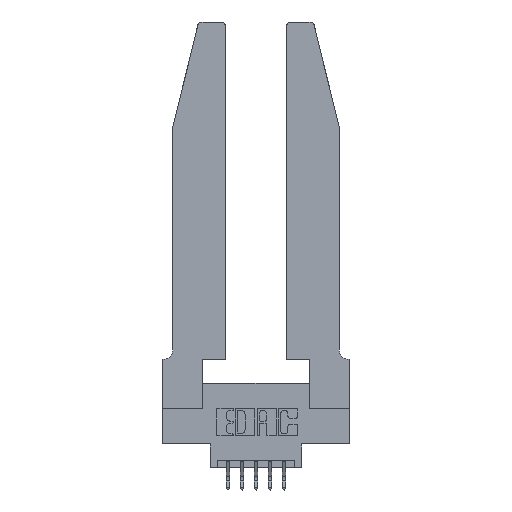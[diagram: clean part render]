
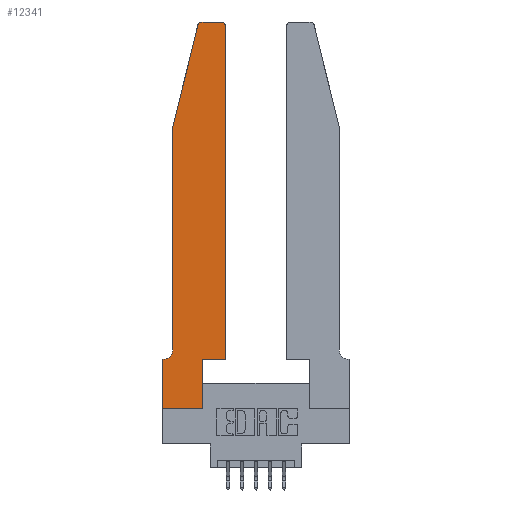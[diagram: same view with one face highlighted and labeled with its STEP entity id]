
A CAD part, top view. The second image highlights one B-rep face of the part: STEP entity #12341.
In plain terms, the highlighted planar face has unit normal (0, 0, 1).
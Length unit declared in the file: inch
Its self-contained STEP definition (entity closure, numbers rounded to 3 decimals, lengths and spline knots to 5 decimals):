
#237 = ORIENTED_EDGE ( 'NONE', *, *, #8766, .T. ) ;
#251 = ORIENTED_EDGE ( 'NONE', *, *, #8956, .T. ) ;
#315 = VERTEX_POINT ( 'NONE', #3736 ) ;
#317 = CARTESIAN_POINT ( 'NONE',  ( 0., 0.35, 0.37 ) ) ;
#403 = CARTESIAN_POINT ( 'NONE',  ( 0.0755, 0.35, 0.37 ) ) ;
#406 = DIRECTION ( 'NONE',  ( -1., 0., 0. ) ) ;
#435 = CARTESIAN_POINT ( 'NONE',  ( 0.4505, 2.72, 0.37 ) ) ;
#501 = CARTESIAN_POINT ( 'NONE',  ( 0., 0., 0.37 ) ) ;
#901 = ORIENTED_EDGE ( 'NONE', *, *, #8134, .T. ) ;
#904 = CARTESIAN_POINT ( 'NONE',  ( 0.0755, 2., 0.37 ) ) ;
#921 = LINE ( 'NONE', #1703, #2313 ) ;
#948 = AXIS2_PLACEMENT_3D ( 'NONE', #317, #1209, #2406 ) ;
#1146 = VERTEX_POINT ( 'NONE', #3767 ) ;
#1209 = DIRECTION ( 'NONE',  ( 0., 0., 1. ) ) ;
#1345 = EDGE_CURVE ( 'NONE', #9358, #4313, #7633, .T. ) ;
#1703 = CARTESIAN_POINT ( 'NONE',  ( 0.4505, 0.35, 0.37 ) ) ;
#1704 = DIRECTION ( 'NONE',  ( 1., 0., 0. ) ) ;
#1751 = DIRECTION ( 'NONE',  ( 0., 0., 1. ) ) ;
#1765 = CARTESIAN_POINT ( 'NONE',  ( 0., 0., 0.37 ) ) ;
#1826 = AXIS2_PLACEMENT_3D ( 'NONE', #13986, #12858, #11785 ) ;
#2122 = VERTEX_POINT ( 'NONE', #435 ) ;
#2232 = ORIENTED_EDGE ( 'NONE', *, *, #6194, .T. ) ;
#2313 = VECTOR ( 'NONE', #7273, 39.37008 ) ;
#2370 = CARTESIAN_POINT ( 'NONE',  ( 0.0755, 2., 0.37 ) ) ;
#2406 = DIRECTION ( 'NONE',  ( 1., 0., 0. ) ) ;
#2489 = CARTESIAN_POINT ( 'NONE',  ( 0.25487, 2.72718, 0.37 ) ) ;
#2533 = EDGE_CURVE ( 'NONE', #315, #7912, #9642, .T. ) ;
#2596 = DIRECTION ( 'NONE',  ( 0., 1., 0. ) ) ;
#2694 = CARTESIAN_POINT ( 'NONE',  ( 0.0055, 0.35, 0.37 ) ) ;
#2858 = DIRECTION ( 'NONE',  ( 0., 0., -1. ) ) ;
#2943 = CARTESIAN_POINT ( 'NONE',  ( 0.2865, 0., 0.37 ) ) ;
#3145 = CIRCLE ( 'NONE', #9103, 0.07 ) ;
#3296 = VECTOR ( 'NONE', #2596, 39.37008 ) ;
#3346 = ORIENTED_EDGE ( 'NONE', *, *, #8570, .T. ) ;
#3736 = CARTESIAN_POINT ( 'NONE',  ( 0.4205, 2.75, 0.37 ) ) ;
#3767 = CARTESIAN_POINT ( 'NONE',  ( 0.4505, 0.35, 0.37 ) ) ;
#3906 = VECTOR ( 'NONE', #5888, 39.37008 ) ;
#4260 = ORIENTED_EDGE ( 'NONE', *, *, #12443, .T. ) ;
#4313 = VERTEX_POINT ( 'NONE', #904 ) ;
#4517 = ORIENTED_EDGE ( 'NONE', *, *, #1345, .T. ) ;
#4708 = CARTESIAN_POINT ( 'NONE',  ( 0.2605, 2.75, 0.37 ) ) ;
#5039 = CARTESIAN_POINT ( 'NONE',  ( 0.2865, 0.35, 0.37 ) ) ;
#5137 = EDGE_LOOP ( 'NONE', ( #7011, #3346, #4517, #4260, #237, #2232, #6688, #901, #13317, #9991, #251, #7016 ) ) ;
#5144 = LINE ( 'NONE', #11391, #11539 ) ;
#5261 = DIRECTION ( 'NONE',  ( 1., 0., 0. ) ) ;
#5613 = LINE ( 'NONE', #11625, #6118 ) ;
#5888 = DIRECTION ( 'NONE',  ( -1., 0., 0. ) ) ;
#6118 = VECTOR ( 'NONE', #9540, 39.37008 ) ;
#6167 = CARTESIAN_POINT ( 'NONE',  ( 0.0055, 0.42, 0.37 ) ) ;
#6194 = EDGE_CURVE ( 'NONE', #7672, #10864, #12871, .T. ) ;
#6222 = DIRECTION ( 'NONE',  ( 1., 0., 0. ) ) ;
#6688 = ORIENTED_EDGE ( 'NONE', *, *, #7036, .T. ) ;
#7011 = ORIENTED_EDGE ( 'NONE', *, *, #2533, .T. ) ;
#7016 = ORIENTED_EDGE ( 'NONE', *, *, #13685, .T. ) ;
#7033 = CARTESIAN_POINT ( 'NONE',  ( 0.4205, 2.72, 0.37 ) ) ;
#7036 = EDGE_CURVE ( 'NONE', #10864, #10337, #5613, .T. ) ;
#7239 = CARTESIAN_POINT ( 'NONE',  ( 0.4505, 0.35, 0.37 ) ) ;
#7273 = DIRECTION ( 'NONE',  ( 0., 1., 0. ) ) ;
#7633 = LINE ( 'NONE', #2370, #8974 ) ;
#7672 = VERTEX_POINT ( 'NONE', #2694 ) ;
#7710 = CARTESIAN_POINT ( 'NONE',  ( 0.0755, 0.42, 0.37 ) ) ;
#7912 = VERTEX_POINT ( 'NONE', #8817 ) ;
#7989 = FACE_OUTER_BOUND ( 'NONE', #5137, .T. ) ;
#8081 = LINE ( 'NONE', #7239, #8582 ) ;
#8134 = EDGE_CURVE ( 'NONE', #10337, #8845, #12133, .T. ) ;
#8429 = VECTOR ( 'NONE', #5261, 39.37008 ) ;
#8570 = EDGE_CURVE ( 'NONE', #7912, #9358, #13137, .T. ) ;
#8582 = VECTOR ( 'NONE', #6222, 39.37008 ) ;
#8671 = CARTESIAN_POINT ( 'NONE',  ( 0., 0.35, 0.37 ) ) ;
#8688 = EDGE_CURVE ( 'NONE', #10714, #1146, #8081, .T. ) ;
#8706 = DIRECTION ( 'NONE',  ( -0.239, -0.971, 0. ) ) ;
#8766 = EDGE_CURVE ( 'NONE', #11622, #7672, #3145, .T. ) ;
#8817 = CARTESIAN_POINT ( 'NONE',  ( 0.284, 2.75, 0.37 ) ) ;
#8845 = VERTEX_POINT ( 'NONE', #2943 ) ;
#8882 = AXIS2_PLACEMENT_3D ( 'NONE', #7033, #1751, #1704 ) ;
#8956 = EDGE_CURVE ( 'NONE', #1146, #2122, #921, .T. ) ;
#8974 = VECTOR ( 'NONE', #8706, 39.37008 ) ;
#9103 = AXIS2_PLACEMENT_3D ( 'NONE', #6167, #2858, #13695 ) ;
#9358 = VERTEX_POINT ( 'NONE', #2489 ) ;
#9540 = DIRECTION ( 'NONE',  ( 0., -1., 0. ) ) ;
#9642 = LINE ( 'NONE', #4708, #11137 ) ;
#9991 = ORIENTED_EDGE ( 'NONE', *, *, #8688, .T. ) ;
#10055 = LINE ( 'NONE', #10195, #3296 ) ;
#10195 = CARTESIAN_POINT ( 'NONE',  ( 0.2865, 0.35, 0.37 ) ) ;
#10235 = DIRECTION ( 'NONE',  ( 0., -1., 0. ) ) ;
#10248 = EDGE_CURVE ( 'NONE', #8845, #10714, #10055, .T. ) ;
#10337 = VERTEX_POINT ( 'NONE', #501 ) ;
#10714 = VERTEX_POINT ( 'NONE', #5039 ) ;
#10864 = VERTEX_POINT ( 'NONE', #8671 ) ;
#11059 = PLANE ( 'NONE',  #948 ) ;
#11137 = VECTOR ( 'NONE', #406, 39.37008 ) ;
#11391 = CARTESIAN_POINT ( 'NONE',  ( 0.0755, 2., 0.37 ) ) ;
#11539 = VECTOR ( 'NONE', #10235, 39.37008 ) ;
#11622 = VERTEX_POINT ( 'NONE', #7710 ) ;
#11625 = CARTESIAN_POINT ( 'NONE',  ( 0., 0., 0.37 ) ) ;
#11785 = DIRECTION ( 'NONE',  ( 1., 0., 0. ) ) ;
#12133 = LINE ( 'NONE', #1765, #8429 ) ;
#12341 = ADVANCED_FACE ( 'NONE', ( #7989 ), #11059, .T. ) ;
#12443 = EDGE_CURVE ( 'NONE', #4313, #11622, #5144, .T. ) ;
#12858 = DIRECTION ( 'NONE',  ( 0., 0., 1. ) ) ;
#12871 = LINE ( 'NONE', #403, #3906 ) ;
#12885 = CIRCLE ( 'NONE', #8882, 0.03 ) ;
#13137 = CIRCLE ( 'NONE', #1826, 0.03 ) ;
#13317 = ORIENTED_EDGE ( 'NONE', *, *, #10248, .T. ) ;
#13685 = EDGE_CURVE ( 'NONE', #2122, #315, #12885, .T. ) ;
#13695 = DIRECTION ( 'NONE',  ( -1., 0., 0. ) ) ;
#13986 = CARTESIAN_POINT ( 'NONE',  ( 0.284, 2.72, 0.37 ) ) ;
